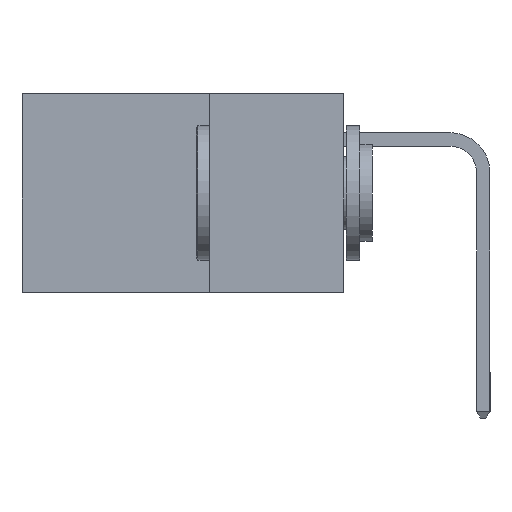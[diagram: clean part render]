
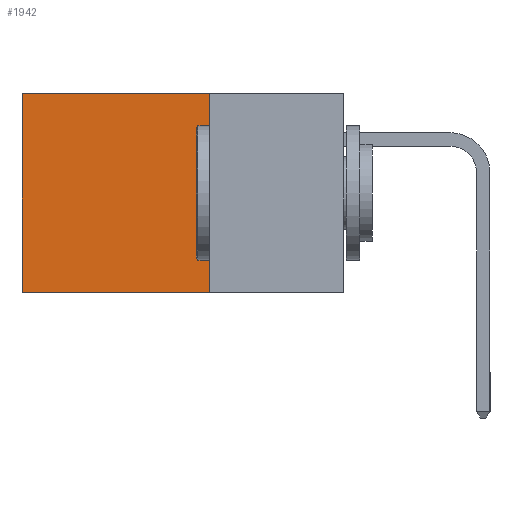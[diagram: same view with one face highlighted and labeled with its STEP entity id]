
A CAD part, left-side view. The second image highlights one B-rep face of the part: STEP entity #1942.
In plain terms, the highlighted planar face has unit normal (-1, 0, 0).
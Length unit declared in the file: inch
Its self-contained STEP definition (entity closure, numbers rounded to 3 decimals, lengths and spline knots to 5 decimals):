
#328 = LINE ( 'NONE', #20895, #10381 ) ;
#337 = CARTESIAN_POINT ( 'NONE',  ( 0.298, 0.25, -0.37 ) ) ;
#860 = VERTEX_POINT ( 'NONE', #20026 ) ;
#1333 = CARTESIAN_POINT ( 'NONE',  ( 0.298, 0.25, 0. ) ) ;
#1550 = LINE ( 'NONE', #8611, #2461 ) ;
#1942 = ADVANCED_FACE ( 'NONE', ( #15335 ), #5582, .F. ) ;
#2461 = VECTOR ( 'NONE', #10285, 39.37008 ) ;
#3412 = EDGE_CURVE ( 'NONE', #23166, #10048, #1550, .T. ) ;
#4567 = CARTESIAN_POINT ( 'NONE',  ( 0.298, 0.6, 0. ) ) ;
#4842 = CARTESIAN_POINT ( 'NONE',  ( 0.298, 0.6, 0. ) ) ;
#4984 = VECTOR ( 'NONE', #10040, 39.37008 ) ;
#5545 = EDGE_CURVE ( 'NONE', #23166, #6435, #328, .T. ) ;
#5582 = PLANE ( 'NONE',  #9463 ) ;
#5587 = LINE ( 'NONE', #21425, #4984 ) ;
#6193 = DIRECTION ( 'NONE',  ( 0., 0., -1. ) ) ;
#6222 = ORIENTED_EDGE ( 'NONE', *, *, #24094, .F. ) ;
#6435 = VERTEX_POINT ( 'NONE', #4842 ) ;
#6619 = DIRECTION ( 'NONE',  ( 0., 0., -1. ) ) ;
#7371 = DIRECTION ( 'NONE',  ( 1., 0., 0. ) ) ;
#7830 = ORIENTED_EDGE ( 'NONE', *, *, #3412, .F. ) ;
#8611 = CARTESIAN_POINT ( 'NONE',  ( 0.298, 0.25, 0. ) ) ;
#9407 = CARTESIAN_POINT ( 'NONE',  ( 0.298, 0.25, 0. ) ) ;
#9463 = AXIS2_PLACEMENT_3D ( 'NONE', #1333, #7371, #6619 ) ;
#10040 = DIRECTION ( 'NONE',  ( 0., 1., 0. ) ) ;
#10048 = VERTEX_POINT ( 'NONE', #337 ) ;
#10285 = DIRECTION ( 'NONE',  ( 0., 0., -1. ) ) ;
#10381 = VECTOR ( 'NONE', #22684, 39.37008 ) ;
#14984 = ORIENTED_EDGE ( 'NONE', *, *, #5545, .T. ) ;
#15335 = FACE_OUTER_BOUND ( 'NONE', #20241, .T. ) ;
#20026 = CARTESIAN_POINT ( 'NONE',  ( 0.298, 0.6, -0.37 ) ) ;
#20241 = EDGE_LOOP ( 'NONE', ( #23207, #6222, #7830, #14984 ) ) ;
#20895 = CARTESIAN_POINT ( 'NONE',  ( 0.298, 0.25, 0. ) ) ;
#21425 = CARTESIAN_POINT ( 'NONE',  ( 0.298, 0.25, -0.37 ) ) ;
#21922 = LINE ( 'NONE', #4567, #22854 ) ;
#22684 = DIRECTION ( 'NONE',  ( 0., 1., 0. ) ) ;
#22854 = VECTOR ( 'NONE', #6193, 39.37008 ) ;
#23166 = VERTEX_POINT ( 'NONE', #9407 ) ;
#23207 = ORIENTED_EDGE ( 'NONE', *, *, #24394, .T. ) ;
#24094 = EDGE_CURVE ( 'NONE', #10048, #860, #5587, .T. ) ;
#24394 = EDGE_CURVE ( 'NONE', #6435, #860, #21922, .T. ) ;
